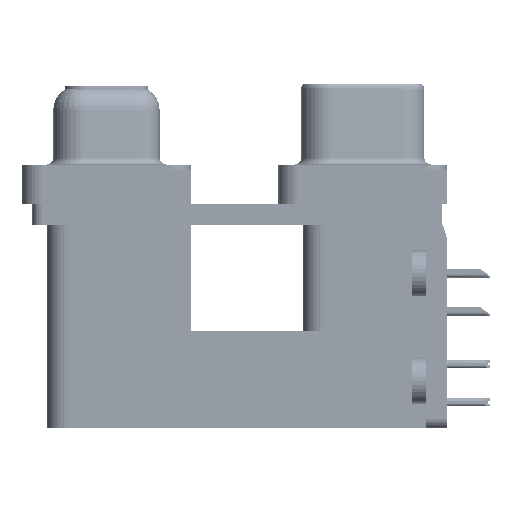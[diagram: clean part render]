
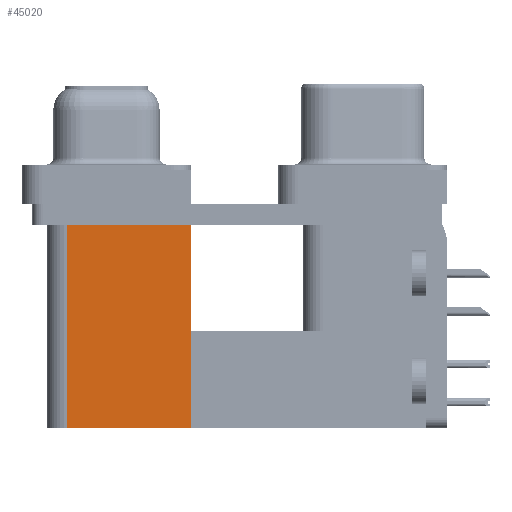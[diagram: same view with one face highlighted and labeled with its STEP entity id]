
A CAD part, left-side view. The second image highlights one B-rep face of the part: STEP entity #45020.
In plain terms, the highlighted planar face has unit normal (-1, 0, 0).
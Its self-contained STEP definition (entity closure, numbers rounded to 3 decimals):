
#50 = CARTESIAN_POINT ( 'NONE',  ( 3.7, 12.775, -19.2 ) ) ;
#4574 = DIRECTION ( 'NONE',  ( 1., 0., 0. ) ) ;
#7123 = EDGE_CURVE ( 'NONE', #48542, #40151, #56024, .T. ) ;
#7579 = DIRECTION ( 'NONE',  ( 0., 0., 1. ) ) ;
#8362 = FACE_OUTER_BOUND ( 'NONE', #29943, .T. ) ;
#8786 = CARTESIAN_POINT ( 'NONE',  ( 3.7, 21.975, -19.2 ) ) ;
#8845 = CARTESIAN_POINT ( 'NONE',  ( 3.7, 21.975, -2.5 ) ) ;
#10907 = ORIENTED_EDGE ( 'NONE', *, *, #7123, .T. ) ;
#11111 = CARTESIAN_POINT ( 'NONE',  ( 3.7, 12.775, -2.5 ) ) ;
#12717 = DIRECTION ( 'NONE',  ( 0., 0., -1. ) ) ;
#13581 = VECTOR ( 'NONE', #33417, 1000. ) ;
#15125 = ORIENTED_EDGE ( 'NONE', *, *, #50856, .F. ) ;
#16032 = EDGE_CURVE ( 'NONE', #40151, #26432, #19522, .T. ) ;
#16567 = CARTESIAN_POINT ( 'NONE',  ( 3.7, 12.775, -19.2 ) ) ;
#17072 = PLANE ( 'NONE',  #31973 ) ;
#17647 = CARTESIAN_POINT ( 'NONE',  ( 3.7, 12.775, -19.2 ) ) ;
#19522 = LINE ( 'NONE', #11111, #45227 ) ;
#23269 = VECTOR ( 'NONE', #7579, 1000. ) ;
#23608 = CARTESIAN_POINT ( 'NONE',  ( 3.7, 21.975, -19.2 ) ) ;
#26432 = VERTEX_POINT ( 'NONE', #8845 ) ;
#27057 = EDGE_CURVE ( 'NONE', #48542, #52161, #36887, .T. ) ;
#27966 = LINE ( 'NONE', #23608, #29499 ) ;
#29499 = VECTOR ( 'NONE', #41333, 1000. ) ;
#29943 = EDGE_LOOP ( 'NONE', ( #48140, #15125, #44150, #10907 ) ) ;
#31973 = AXIS2_PLACEMENT_3D ( 'NONE', #17647, #4574, #12717 ) ;
#33417 = DIRECTION ( 'NONE',  ( 0., 1., 0. ) ) ;
#33684 = CARTESIAN_POINT ( 'NONE',  ( 3.7, 12.775, -2.5 ) ) ;
#36887 = LINE ( 'NONE', #50817, #13581 ) ;
#40151 = VERTEX_POINT ( 'NONE', #33684 ) ;
#41333 = DIRECTION ( 'NONE',  ( 0., 0., 1. ) ) ;
#44150 = ORIENTED_EDGE ( 'NONE', *, *, #27057, .F. ) ;
#45020 = ADVANCED_FACE ( 'NONE', ( #8362 ), #17072, .F. ) ;
#45227 = VECTOR ( 'NONE', #46488, 1000. ) ;
#46488 = DIRECTION ( 'NONE',  ( 0., 1., 0. ) ) ;
#48140 = ORIENTED_EDGE ( 'NONE', *, *, #16032, .T. ) ;
#48542 = VERTEX_POINT ( 'NONE', #50 ) ;
#50817 = CARTESIAN_POINT ( 'NONE',  ( 3.7, 12.775, -19.2 ) ) ;
#50856 = EDGE_CURVE ( 'NONE', #52161, #26432, #27966, .T. ) ;
#52161 = VERTEX_POINT ( 'NONE', #8786 ) ;
#56024 = LINE ( 'NONE', #16567, #23269 ) ;
